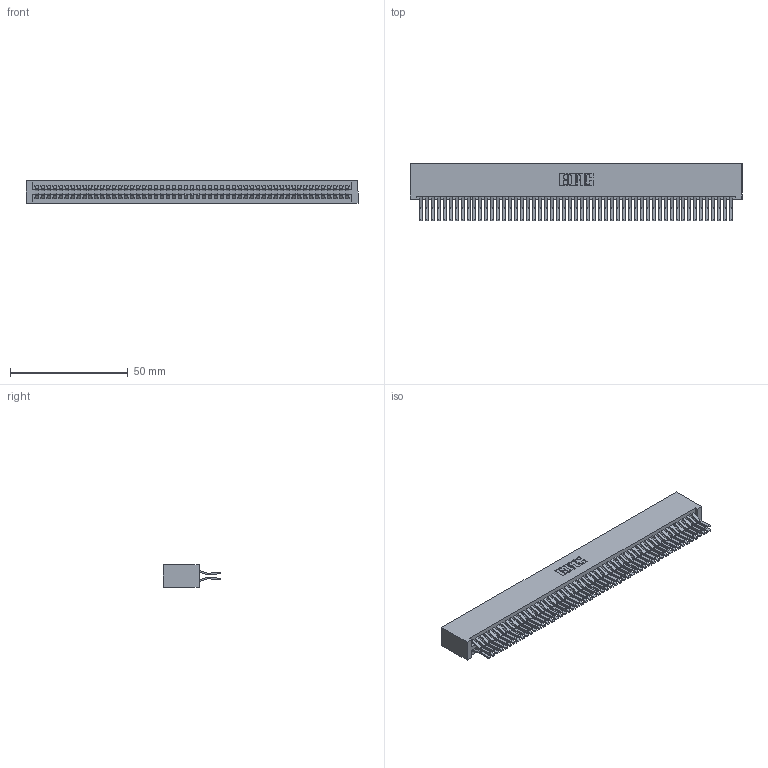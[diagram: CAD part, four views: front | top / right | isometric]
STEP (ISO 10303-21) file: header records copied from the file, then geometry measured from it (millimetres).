
FILE_DESCRIPTION (( 'STEP AP203' ), '1' );
FILE_NAME ('345-106-560-201.STEP', '2018-10-07T04:19:30', ( '' ), ( '' ), 'SwSTEP 2.0', 'SolidWorks 2016', '' );
FILE_SCHEMA (( 'CONFIG_CONTROL_DESIGN' ));
Length unit declared in the file: inch
Products named in the file (3): 345-292-001_560 Tail; 345-106-560-201; 345 Part_No Mounting Lugs
Assembly tree (111 placements, depth 2):
  345-106-560-201
    345 Part_No Mounting Lugs
    345-292-001_560 Tail  x106
Bounding box: 141.22 x 24.45 x 9.4 mm (x, y, z)
Volume: 15131.4 mm3; surface area: 24670.1 mm2
Topology: 107 solids, 107 shells, 5630 faces, 16747 edges, 11022 vertices
Faces by surface type: plane 3574, cylinder 2056
Entity records: 39919 total; most frequent: CARTESIAN_POINT 6680, ORIENTED_EDGE 6614, DIRECTION 5875, EDGE_CURVE 3307, LINE 2967, VECTOR 2967, VERTEX_POINT 2202, AXIS2_PLACEMENT_3D 1454
